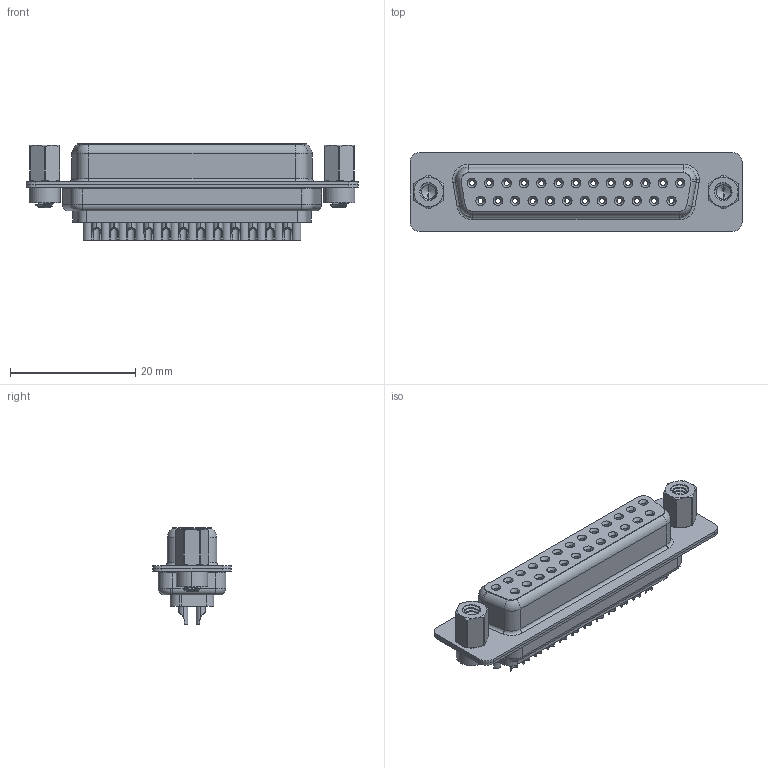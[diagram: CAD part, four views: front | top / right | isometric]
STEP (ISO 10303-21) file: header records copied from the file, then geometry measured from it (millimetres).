
FILE_DESCRIPTION (( 'STEP AP203' ), '1' );
FILE_NAME ('628-025-322-043.STEP', '2020-07-14T13:47:18', ( '' ), ( '' ), 'SwSTEP 2.0', 'SolidWorks 2020', '' );
FILE_SCHEMA (( 'CONFIG_CONTROL_DESIGN' ));
Length unit declared in the file: millimetre
Products named in the file (8): 628 Contact Row 1_22L; 628 4-40 Threaded Rivet; 628 Housing_25 LP; 628 Contact Row 2_22L; 628-025-322-043; 628 Shell Rear_25 Contacts; 628 Shell Front_25 Contacts; 628 4-40 Hex Standoff
Assembly tree (32 placements, depth 2):
  628-025-322-043
    628 Housing_25 LP
    628 Shell Front_25 Contacts
    628 Shell Rear_25 Contacts
    628 Contact Row 1_22L  x13
    628 Contact Row 2_22L  x12
    628 4-40 Threaded Rivet  x2
    628 4-40 Hex Standoff  x2
Bounding box: 53 x 12.6 x 15.35 mm (x, y, z)
Volume: 4052 mm3; surface area: 9862.1 mm2
Topology: 32 solids, 32 shells, 2626 faces, 6673 edges, 4197 vertices
Faces by surface type: cylinder 832, plane 614, bspline 518, torus 507, cone 155
Entity records: 30107 total; most frequent: CARTESIAN_POINT 10311, DIRECTION 3977, ORIENTED_EDGE 3734, EDGE_CURVE 1867, AXIS2_PLACEMENT_3D 1660, VERTEX_POINT 1183, EDGE_LOOP 934, CIRCLE 890
